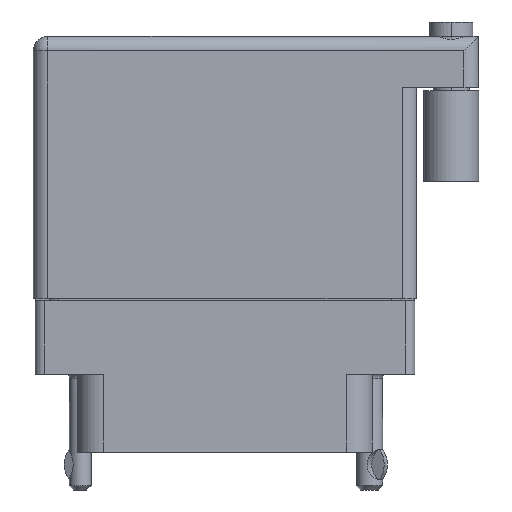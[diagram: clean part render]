
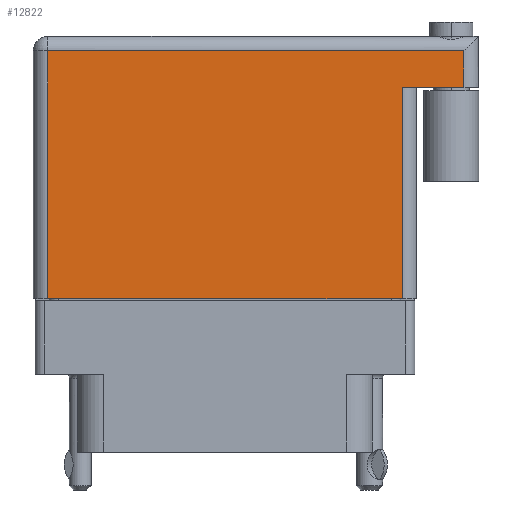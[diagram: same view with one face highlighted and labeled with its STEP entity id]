
A CAD part, front view. The second image highlights one B-rep face of the part: STEP entity #12822.
In plain terms, the highlighted face is planar.
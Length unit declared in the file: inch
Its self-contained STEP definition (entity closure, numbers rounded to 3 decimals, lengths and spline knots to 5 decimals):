
#1418 = ORIENTED_EDGE ( 'NONE', *, *, #23680, .F. ) ;
#2103 = CARTESIAN_POINT ( 'NONE',  ( 0.6125, 0.631, 0.3575 ) ) ;
#2488 = PLANE ( 'NONE',  #4733 ) ;
#2679 = DIRECTION ( 'NONE',  ( -1., 0., 0. ) ) ;
#2879 = VECTOR ( 'NONE', #14238, 39.37008 ) ;
#3339 = LINE ( 'NONE', #21109, #18626 ) ;
#3741 = VERTEX_POINT ( 'NONE', #28427 ) ;
#4091 = EDGE_LOOP ( 'NONE', ( #13711, #29405, #1418, #17266, #11968, #10644 ) ) ;
#4733 = AXIS2_PLACEMENT_3D ( 'NONE', #5698, #14776, #2679 ) ;
#4917 = EDGE_CURVE ( 'NONE', #11137, #7972, #34357, .T. ) ;
#5698 = CARTESIAN_POINT ( 'NONE',  ( -0.6625, 0.806, 0.3575 ) ) ;
#7414 = EDGE_CURVE ( 'NONE', #10591, #35390, #26360, .T. ) ;
#7850 = CARTESIAN_POINT ( 'NONE',  ( 0.8265, 0.756, 0.3575 ) ) ;
#7972 = VERTEX_POINT ( 'NONE', #2103 ) ;
#9712 = CARTESIAN_POINT ( 'NONE',  ( 0.6125, 0.631, 0.3575 ) ) ;
#10591 = VERTEX_POINT ( 'NONE', #35677 ) ;
#10644 = ORIENTED_EDGE ( 'NONE', *, *, #38054, .T. ) ;
#11137 = VERTEX_POINT ( 'NONE', #37004 ) ;
#11968 = ORIENTED_EDGE ( 'NONE', *, *, #33799, .T. ) ;
#12242 = DIRECTION ( 'NONE',  ( 1., 0., 0. ) ) ;
#12326 = DIRECTION ( 'NONE',  ( 0., 1., 0. ) ) ;
#12822 = ADVANCED_FACE ( 'NONE', ( #21039 ), #2488, .F. ) ;
#13668 = VERTEX_POINT ( 'NONE', #35974 ) ;
#13711 = ORIENTED_EDGE ( 'NONE', *, *, #20994, .T. ) ;
#14238 = DIRECTION ( 'NONE',  ( 0., 1., 0. ) ) ;
#14776 = DIRECTION ( 'NONE',  ( 0., 0., -1. ) ) ;
#15186 = CARTESIAN_POINT ( 'NONE',  ( 0.8765, 0.631, 0.3575 ) ) ;
#17266 = ORIENTED_EDGE ( 'NONE', *, *, #7414, .T. ) ;
#17870 = VECTOR ( 'NONE', #36614, 39.37008 ) ;
#18626 = VECTOR ( 'NONE', #33624, 39.37008 ) ;
#20994 = EDGE_CURVE ( 'NONE', #3741, #11137, #27590, .T. ) ;
#21039 = FACE_OUTER_BOUND ( 'NONE', #4091, .T. ) ;
#21109 = CARTESIAN_POINT ( 'NONE',  ( -0.6125, -0.1, 0.3575 ) ) ;
#23680 = EDGE_CURVE ( 'NONE', #10591, #7972, #33575, .T. ) ;
#24132 = CARTESIAN_POINT ( 'NONE',  ( 0.8265, 0.806, 0.3575 ) ) ;
#24485 = DIRECTION ( 'NONE',  ( -1., 0., 0. ) ) ;
#26360 = LINE ( 'NONE', #24132, #2879 ) ;
#27590 = LINE ( 'NONE', #34263, #29679 ) ;
#28427 = CARTESIAN_POINT ( 'NONE',  ( -0.6125, -0.1, 0.3575 ) ) ;
#28583 = LINE ( 'NONE', #29945, #17870 ) ;
#29405 = ORIENTED_EDGE ( 'NONE', *, *, #4917, .T. ) ;
#29679 = VECTOR ( 'NONE', #12242, 39.37008 ) ;
#29945 = CARTESIAN_POINT ( 'NONE',  ( -0.6625, 0.756, 0.3575 ) ) ;
#33575 = LINE ( 'NONE', #15186, #37270 ) ;
#33624 = DIRECTION ( 'NONE',  ( 0., -1., 0. ) ) ;
#33799 = EDGE_CURVE ( 'NONE', #35390, #13668, #28583, .T. ) ;
#34263 = CARTESIAN_POINT ( 'NONE',  ( -0.6625, -0.1, 0.3575 ) ) ;
#34357 = LINE ( 'NONE', #9712, #35749 ) ;
#35390 = VERTEX_POINT ( 'NONE', #7850 ) ;
#35677 = CARTESIAN_POINT ( 'NONE',  ( 0.8265, 0.631, 0.3575 ) ) ;
#35749 = VECTOR ( 'NONE', #12326, 39.37008 ) ;
#35974 = CARTESIAN_POINT ( 'NONE',  ( -0.6125, 0.756, 0.3575 ) ) ;
#36614 = DIRECTION ( 'NONE',  ( -1., 0., 0. ) ) ;
#37004 = CARTESIAN_POINT ( 'NONE',  ( 0.6125, -0.1, 0.3575 ) ) ;
#37270 = VECTOR ( 'NONE', #24485, 39.37008 ) ;
#38054 = EDGE_CURVE ( 'NONE', #13668, #3741, #3339, .T. ) ;
